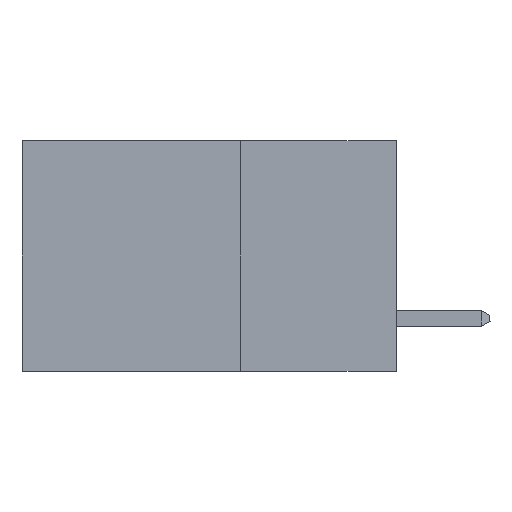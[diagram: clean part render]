
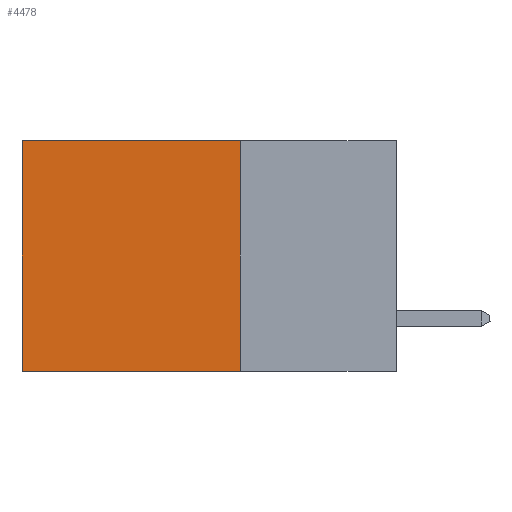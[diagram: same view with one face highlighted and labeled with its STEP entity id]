
A CAD part, left-side view. The second image highlights one B-rep face of the part: STEP entity #4478.
In plain terms, the highlighted planar face has unit normal (-1, 0, 0).
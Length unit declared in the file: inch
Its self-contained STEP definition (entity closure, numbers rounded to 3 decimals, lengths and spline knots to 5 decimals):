
#553 = DIRECTION ( 'NONE',  ( 0., 1., 0. ) ) ;
#2197 = ORIENTED_EDGE ( 'NONE', *, *, #6682, .T. ) ;
#2242 = VERTEX_POINT ( 'NONE', #10074 ) ;
#2646 = DIRECTION ( 'NONE',  ( 0., 0., -1. ) ) ;
#2649 = EDGE_CURVE ( 'NONE', #4031, #8744, #6753, .T. ) ;
#2679 = CARTESIAN_POINT ( 'NONE',  ( 0.298, 0.25, 0. ) ) ;
#2706 = CARTESIAN_POINT ( 'NONE',  ( 0.298, 0.25, 0. ) ) ;
#3231 = ORIENTED_EDGE ( 'NONE', *, *, #2649, .T. ) ;
#3535 = LINE ( 'NONE', #2679, #4317 ) ;
#3811 = CARTESIAN_POINT ( 'NONE',  ( 0.298, 0.6, 0. ) ) ;
#3930 = DIRECTION ( 'NONE',  ( 0., 0., -1. ) ) ;
#4031 = VERTEX_POINT ( 'NONE', #3811 ) ;
#4317 = VECTOR ( 'NONE', #2646, 39.37008 ) ;
#4410 = ORIENTED_EDGE ( 'NONE', *, *, #9515, .F. ) ;
#4478 = ADVANCED_FACE ( 'NONE', ( #6973 ), #7792, .F. ) ;
#4550 = CARTESIAN_POINT ( 'NONE',  ( 0.298, 0.25, -0.37 ) ) ;
#4800 = EDGE_LOOP ( 'NONE', ( #3231, #4410, #10583, #2197 ) ) ;
#5188 = AXIS2_PLACEMENT_3D ( 'NONE', #2706, #6190, #10319 ) ;
#5499 = VECTOR ( 'NONE', #553, 39.37008 ) ;
#5568 = LINE ( 'NONE', #4550, #8604 ) ;
#5592 = CARTESIAN_POINT ( 'NONE',  ( 0.298, 0.6, 0. ) ) ;
#5600 = CARTESIAN_POINT ( 'NONE',  ( 0.298, 0.25, 0. ) ) ;
#6190 = DIRECTION ( 'NONE',  ( 1., 0., 0. ) ) ;
#6356 = CARTESIAN_POINT ( 'NONE',  ( 0.298, 0.6, -0.37 ) ) ;
#6453 = EDGE_CURVE ( 'NONE', #2242, #7206, #3535, .T. ) ;
#6682 = EDGE_CURVE ( 'NONE', #2242, #4031, #8788, .T. ) ;
#6753 = LINE ( 'NONE', #5592, #7254 ) ;
#6973 = FACE_OUTER_BOUND ( 'NONE', #4800, .T. ) ;
#7206 = VERTEX_POINT ( 'NONE', #7698 ) ;
#7254 = VECTOR ( 'NONE', #3930, 39.37008 ) ;
#7698 = CARTESIAN_POINT ( 'NONE',  ( 0.298, 0.25, -0.37 ) ) ;
#7792 = PLANE ( 'NONE',  #5188 ) ;
#8604 = VECTOR ( 'NONE', #8614, 39.37008 ) ;
#8614 = DIRECTION ( 'NONE',  ( 0., 1., 0. ) ) ;
#8744 = VERTEX_POINT ( 'NONE', #6356 ) ;
#8788 = LINE ( 'NONE', #5600, #5499 ) ;
#9515 = EDGE_CURVE ( 'NONE', #7206, #8744, #5568, .T. ) ;
#10074 = CARTESIAN_POINT ( 'NONE',  ( 0.298, 0.25, 0. ) ) ;
#10319 = DIRECTION ( 'NONE',  ( 0., 0., -1. ) ) ;
#10583 = ORIENTED_EDGE ( 'NONE', *, *, #6453, .F. ) ;
